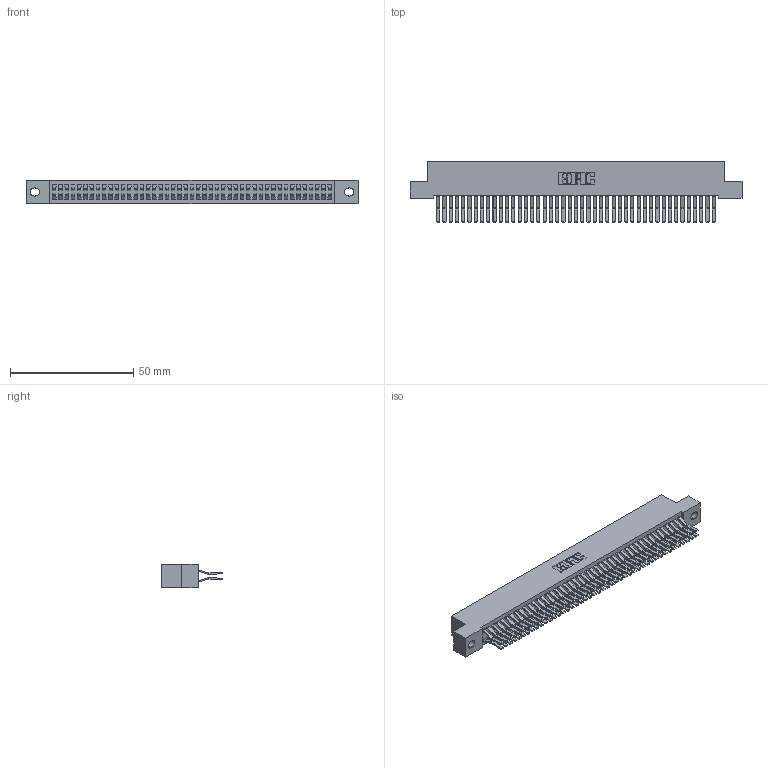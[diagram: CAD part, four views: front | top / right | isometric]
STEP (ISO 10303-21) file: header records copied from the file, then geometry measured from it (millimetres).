
FILE_DESCRIPTION (( 'STEP AP203' ), '1' );
FILE_NAME ('392-090-560-202.STEP', '2018-08-18T07:32:20', ( '' ), ( '' ), 'SwSTEP 2.0', 'SolidWorks 2016', '' );
FILE_SCHEMA (( 'CONFIG_CONTROL_DESIGN' ));
Length unit declared in the file: inch
Products named in the file (3): 342 Part_.128 Slot; 345-292-001_560 Tail; 392-090-560-202
Assembly tree (91 placements, depth 2):
  392-090-560-202
    342 Part_.128 Slot
    345-292-001_560 Tail  x90
Bounding box: 134.62 x 24.78 x 9.4 mm (x, y, z)
Volume: 12648.5 mm3; surface area: 21838.9 mm2
Topology: 91 solids, 91 shells, 4974 faces, 14801 edges, 9746 vertices
Faces by surface type: plane 3310, cylinder 1664
Entity records: 28653 total; most frequent: CARTESIAN_POINT 4746, ORIENTED_EDGE 4682, DIRECTION 4053, EDGE_CURVE 2341, VECTOR 2209, LINE 2209, VERTEX_POINT 1558, AXIS2_PLACEMENT_3D 922
